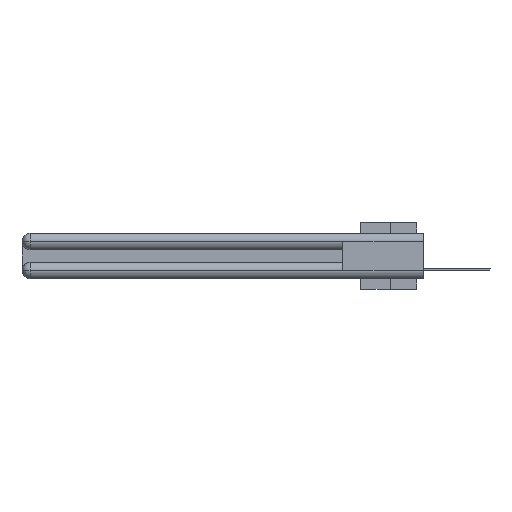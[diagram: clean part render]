
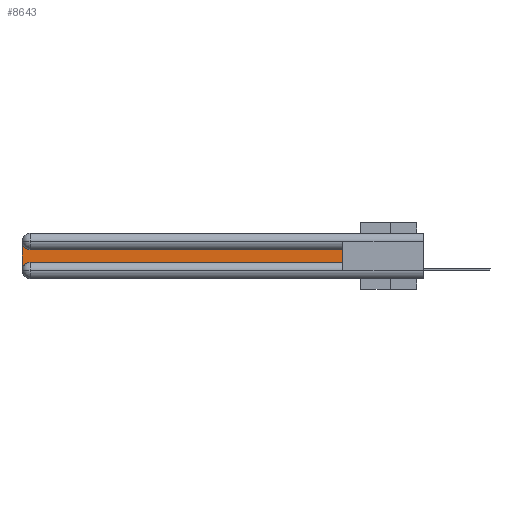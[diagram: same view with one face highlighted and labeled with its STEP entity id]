
A CAD part, left-side view. The second image highlights one B-rep face of the part: STEP entity #8643.
In plain terms, the highlighted planar face has unit normal (-1, 0, 0).
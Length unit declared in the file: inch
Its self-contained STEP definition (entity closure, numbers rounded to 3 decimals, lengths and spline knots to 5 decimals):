
#969 = VERTEX_POINT ( 'NONE', #7673 ) ;
#1077 = CARTESIAN_POINT ( 'NONE',  ( 0.075, 3., -0.1225 ) ) ;
#1186 = CARTESIAN_POINT ( 'NONE',  ( 0.075, 2.94, -0.0625 ) ) ;
#1556 = DIRECTION ( 'NONE',  ( 0., 0., 1. ) ) ;
#1789 = EDGE_CURVE ( 'NONE', #33763, #24552, #15094, .T. ) ;
#2006 = CARTESIAN_POINT ( 'NONE',  ( 0.075, 2.94, -0.2775 ) ) ;
#3853 = CARTESIAN_POINT ( 'NONE',  ( 0.075, 2.94, -0.1225 ) ) ;
#3899 = VECTOR ( 'NONE', #1556, 39.37008 ) ;
#6958 = ORIENTED_EDGE ( 'NONE', *, *, #32905, .T. ) ;
#7248 = CIRCLE ( 'NONE', #32410, 0.06 ) ;
#7673 = CARTESIAN_POINT ( 'NONE',  ( 0.075, 3., -0.0625 ) ) ;
#8510 = ORIENTED_EDGE ( 'NONE', *, *, #10396, .T. ) ;
#8643 = ADVANCED_FACE ( 'NONE', ( #9245 ), #8803, .F. ) ;
#8803 = PLANE ( 'NONE',  #20406 ) ;
#9245 = FACE_OUTER_BOUND ( 'NONE', #25032, .T. ) ;
#9743 = DIRECTION ( 'NONE',  ( 1., 0., 0. ) ) ;
#10219 = DIRECTION ( 'NONE',  ( 0., -1., 0. ) ) ;
#10396 = EDGE_CURVE ( 'NONE', #20047, #33763, #32660, .T. ) ;
#10741 = VECTOR ( 'NONE', #10219, 39.37008 ) ;
#10932 = ORIENTED_EDGE ( 'NONE', *, *, #19911, .T. ) ;
#14081 = CIRCLE ( 'NONE', #15083, 0.06 ) ;
#14321 = LINE ( 'NONE', #16749, #32083 ) ;
#14967 = EDGE_CURVE ( 'NONE', #23424, #969, #7248, .T. ) ;
#15083 = AXIS2_PLACEMENT_3D ( 'NONE', #2006, #9743, #28248 ) ;
#15094 = LINE ( 'NONE', #31102, #3899 ) ;
#15827 = ORIENTED_EDGE ( 'NONE', *, *, #14967, .T. ) ;
#16542 = DIRECTION ( 'NONE',  ( 1., 0., 0. ) ) ;
#16749 = CARTESIAN_POINT ( 'NONE',  ( 0.075, 0.6, -0.1225 ) ) ;
#17734 = DIRECTION ( 'NONE',  ( 0., 0., -1. ) ) ;
#19048 = VECTOR ( 'NONE', #17734, 39.37008 ) ;
#19624 = DIRECTION ( 'NONE',  ( 1., 0., 0. ) ) ;
#19911 = EDGE_CURVE ( 'NONE', #969, #24701, #26100, .T. ) ;
#20047 = VERTEX_POINT ( 'NONE', #21166 ) ;
#20221 = ORIENTED_EDGE ( 'NONE', *, *, #1789, .T. ) ;
#20406 = AXIS2_PLACEMENT_3D ( 'NONE', #1077, #16542, #29964 ) ;
#21166 = CARTESIAN_POINT ( 'NONE',  ( 0.075, 2.94, -0.2175 ) ) ;
#22302 = DIRECTION ( 'NONE',  ( 0., 0., -1. ) ) ;
#23329 = CARTESIAN_POINT ( 'NONE',  ( 0.075, 0.6, -0.2175 ) ) ;
#23424 = VERTEX_POINT ( 'NONE', #3853 ) ;
#24552 = VERTEX_POINT ( 'NONE', #27037 ) ;
#24701 = VERTEX_POINT ( 'NONE', #24978 ) ;
#24978 = CARTESIAN_POINT ( 'NONE',  ( 0.075, 3., -0.2775 ) ) ;
#25032 = EDGE_LOOP ( 'NONE', ( #6958, #15827, #10932, #28606, #8510, #20221 ) ) ;
#26050 = CARTESIAN_POINT ( 'NONE',  ( 0.075, 0.6, -0.2175 ) ) ;
#26100 = LINE ( 'NONE', #28401, #19048 ) ;
#27037 = CARTESIAN_POINT ( 'NONE',  ( 0.075, 0.6, -0.1225 ) ) ;
#28248 = DIRECTION ( 'NONE',  ( 0., 0., -1. ) ) ;
#28401 = CARTESIAN_POINT ( 'NONE',  ( 0.075, 3., -0.2175 ) ) ;
#28606 = ORIENTED_EDGE ( 'NONE', *, *, #30631, .T. ) ;
#29964 = DIRECTION ( 'NONE',  ( 0., 0., -1. ) ) ;
#30631 = EDGE_CURVE ( 'NONE', #24701, #20047, #14081, .T. ) ;
#31102 = CARTESIAN_POINT ( 'NONE',  ( 0.075, 0.6, -0.2175 ) ) ;
#32083 = VECTOR ( 'NONE', #33039, 39.37008 ) ;
#32410 = AXIS2_PLACEMENT_3D ( 'NONE', #1186, #19624, #22302 ) ;
#32660 = LINE ( 'NONE', #26050, #10741 ) ;
#32905 = EDGE_CURVE ( 'NONE', #24552, #23424, #14321, .T. ) ;
#33039 = DIRECTION ( 'NONE',  ( 0., 1., 0. ) ) ;
#33763 = VERTEX_POINT ( 'NONE', #23329 ) ;
